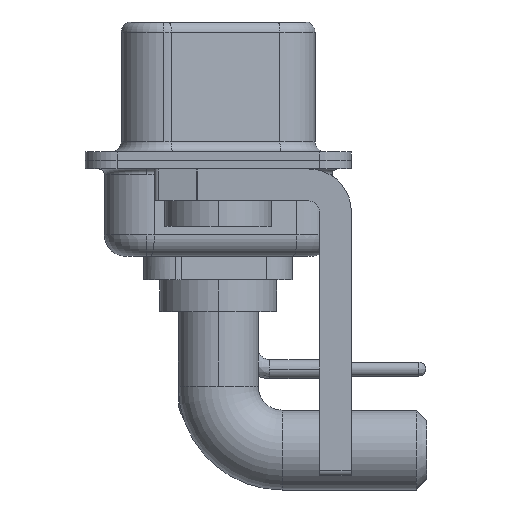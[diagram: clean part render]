
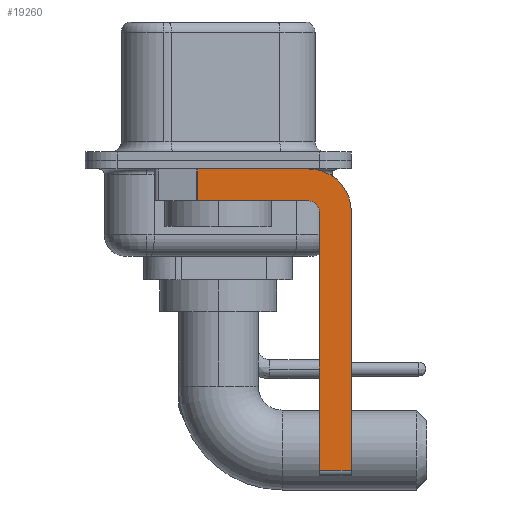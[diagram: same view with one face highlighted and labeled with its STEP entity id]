
A CAD part, left-side view. The second image highlights one B-rep face of the part: STEP entity #19260.
In plain terms, the highlighted planar face has unit normal (-1, 0, 0).
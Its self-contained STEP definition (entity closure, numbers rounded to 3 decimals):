
#35 = VERTEX_POINT ( 'NONE', #5579 ) ;
#174 = AXIS2_PLACEMENT_3D ( 'NONE', #6742, #3040, #12686 ) ;
#656 = EDGE_CURVE ( 'NONE', #24234, #5296, #12454, .T. ) ;
#711 = CARTESIAN_POINT ( 'NONE',  ( -2.9, -4.25, -14.55 ) ) ;
#898 = LINE ( 'NONE', #21615, #15753 ) ;
#1040 = VERTEX_POINT ( 'NONE', #23347 ) ;
#1188 = EDGE_CURVE ( 'NONE', #7292, #22814, #21489, .T. ) ;
#1485 = AXIS2_PLACEMENT_3D ( 'NONE', #12604, #5160, #12839 ) ;
#2119 = CARTESIAN_POINT ( 'NONE',  ( -2.9, -6.25, -2.4 ) ) ;
#3040 = DIRECTION ( 'NONE',  ( 1., 0., 0. ) ) ;
#3448 = ORIENTED_EDGE ( 'NONE', *, *, #17907, .T. ) ;
#3716 = ORIENTED_EDGE ( 'NONE', *, *, #17938, .F. ) ;
#3948 = CARTESIAN_POINT ( 'NONE',  ( -2.9, -6.25, -2.4 ) ) ;
#4253 = DIRECTION ( 'NONE',  ( 0., -1., 0. ) ) ;
#4486 = DIRECTION ( 'NONE',  ( 0., 0., -1. ) ) ;
#4912 = DIRECTION ( 'NONE',  ( 0., 0., 1. ) ) ;
#4961 = ORIENTED_EDGE ( 'NONE', *, *, #16269, .F. ) ;
#5160 = DIRECTION ( 'NONE',  ( 1., 0., 0. ) ) ;
#5296 = VERTEX_POINT ( 'NONE', #2119 ) ;
#5304 = VECTOR ( 'NONE', #12739, 1000. ) ;
#5455 = CARTESIAN_POINT ( 'NONE',  ( -2.9, 0.978, -0.4 ) ) ;
#5579 = CARTESIAN_POINT ( 'NONE',  ( -2.9, -6.25, -14.55 ) ) ;
#6137 = VECTOR ( 'NONE', #4486, 1000. ) ;
#6674 = ORIENTED_EDGE ( 'NONE', *, *, #20292, .F. ) ;
#6742 = CARTESIAN_POINT ( 'NONE',  ( -2.9, -4.25, -2.4 ) ) ;
#6896 = DIRECTION ( 'NONE',  ( -1., 0., 0. ) ) ;
#6919 = LINE ( 'NONE', #15973, #5304 ) ;
#6964 = AXIS2_PLACEMENT_3D ( 'NONE', #18538, #6896, #4912 ) ;
#7122 = VERTEX_POINT ( 'NONE', #21839 ) ;
#7292 = VERTEX_POINT ( 'NONE', #5455 ) ;
#7536 = CARTESIAN_POINT ( 'NONE',  ( -2.9, 0.978, -1.9 ) ) ;
#8234 = CARTESIAN_POINT ( 'NONE',  ( -2.9, -4.25, -0.4 ) ) ;
#10742 = ORIENTED_EDGE ( 'NONE', *, *, #656, .F. ) ;
#11625 = EDGE_LOOP ( 'NONE', ( #21660, #15231, #4961, #3716, #21899, #3448, #6674, #10742 ) ) ;
#12123 = CARTESIAN_POINT ( 'NONE',  ( -2.9, -4.25, -1.9 ) ) ;
#12454 = CIRCLE ( 'NONE', #174, 2. ) ;
#12604 = CARTESIAN_POINT ( 'NONE',  ( -2.9, -4.25, -2.4 ) ) ;
#12686 = DIRECTION ( 'NONE',  ( 0., 0., -1. ) ) ;
#12739 = DIRECTION ( 'NONE',  ( 0., 0., 1. ) ) ;
#12839 = DIRECTION ( 'NONE',  ( 0., 0., -1. ) ) ;
#13184 = DIRECTION ( 'NONE',  ( 0., 1., 0. ) ) ;
#13425 = VERTEX_POINT ( 'NONE', #12123 ) ;
#14437 = EDGE_CURVE ( 'NONE', #7122, #1040, #6919, .T. ) ;
#15048 = CARTESIAN_POINT ( 'NONE',  ( -2.9, -4.25, -1.9 ) ) ;
#15231 = ORIENTED_EDGE ( 'NONE', *, *, #1188, .T. ) ;
#15753 = VECTOR ( 'NONE', #4253, 1000. ) ;
#15973 = CARTESIAN_POINT ( 'NONE',  ( -2.9, -4.75, -14.8 ) ) ;
#16269 = EDGE_CURVE ( 'NONE', #13425, #22814, #22504, .T. ) ;
#16963 = VECTOR ( 'NONE', #23039, 1000. ) ;
#17560 = DIRECTION ( 'NONE',  ( 0., -1., 0. ) ) ;
#17689 = LINE ( 'NONE', #711, #23185 ) ;
#17907 = EDGE_CURVE ( 'NONE', #7122, #35, #17689, .T. ) ;
#17938 = EDGE_CURVE ( 'NONE', #1040, #13425, #18447, .T. ) ;
#17974 = VECTOR ( 'NONE', #13184, 1000. ) ;
#18447 = CIRCLE ( 'NONE', #6964, 0.5 ) ;
#18538 = CARTESIAN_POINT ( 'NONE',  ( -2.9, -4.25, -2.4 ) ) ;
#19260 = ADVANCED_FACE ( 'NONE', ( #23902 ), #20407, .F. ) ;
#19428 = LINE ( 'NONE', #3948, #16963 ) ;
#20044 = EDGE_CURVE ( 'NONE', #7292, #24234, #898, .T. ) ;
#20292 = EDGE_CURVE ( 'NONE', #5296, #35, #19428, .T. ) ;
#20407 = PLANE ( 'NONE',  #1485 ) ;
#21489 = LINE ( 'NONE', #23599, #6137 ) ;
#21615 = CARTESIAN_POINT ( 'NONE',  ( -2.9, 3., -0.4 ) ) ;
#21660 = ORIENTED_EDGE ( 'NONE', *, *, #20044, .F. ) ;
#21839 = CARTESIAN_POINT ( 'NONE',  ( -2.9, -4.75, -14.55 ) ) ;
#21899 = ORIENTED_EDGE ( 'NONE', *, *, #14437, .F. ) ;
#22504 = LINE ( 'NONE', #15048, #17974 ) ;
#22814 = VERTEX_POINT ( 'NONE', #7536 ) ;
#23039 = DIRECTION ( 'NONE',  ( 0., 0., -1. ) ) ;
#23185 = VECTOR ( 'NONE', #17560, 1000. ) ;
#23347 = CARTESIAN_POINT ( 'NONE',  ( -2.9, -4.75, -2.4 ) ) ;
#23599 = CARTESIAN_POINT ( 'NONE',  ( -2.9, 0.978, -1.9 ) ) ;
#23902 = FACE_OUTER_BOUND ( 'NONE', #11625, .T. ) ;
#24234 = VERTEX_POINT ( 'NONE', #8234 ) ;
